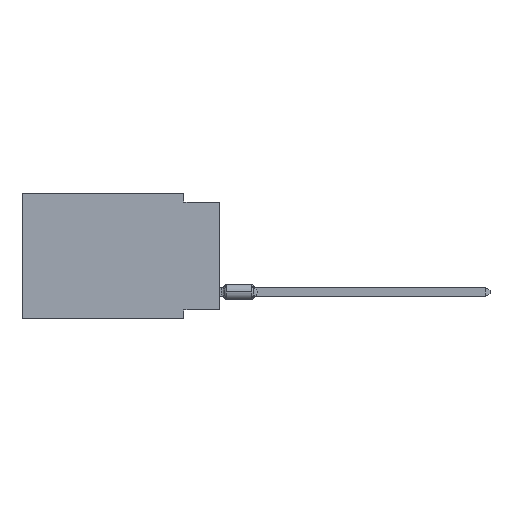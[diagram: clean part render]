
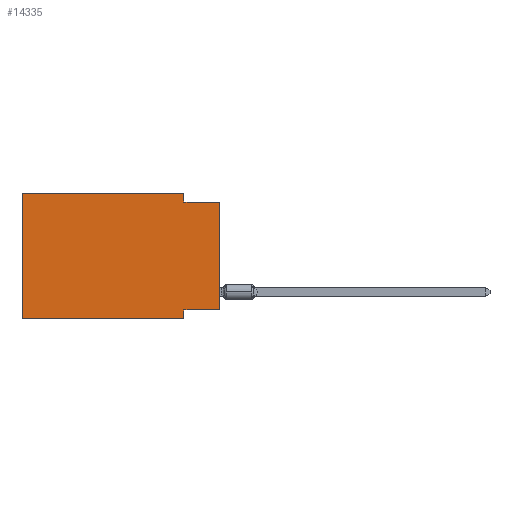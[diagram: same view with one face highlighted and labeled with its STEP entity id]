
A CAD part, left-side view. The second image highlights one B-rep face of the part: STEP entity #14335.
In plain terms, the highlighted planar face has unit normal (-1, 0, 0).
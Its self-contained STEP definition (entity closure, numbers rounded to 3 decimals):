
#148 = VECTOR ( 'NONE', #24377, 1000. ) ;
#185 = VECTOR ( 'NONE', #12506, 1000. ) ;
#1087 = DIRECTION ( 'NONE',  ( 1., 0., 0. ) ) ;
#1091 = ORIENTED_EDGE ( 'NONE', *, *, #11967, .F. ) ;
#1568 = EDGE_CURVE ( 'NONE', #18166, #24625, #8059, .T. ) ;
#1662 = ORIENTED_EDGE ( 'NONE', *, *, #21237, .T. ) ;
#1938 = ORIENTED_EDGE ( 'NONE', *, *, #7770, .F. ) ;
#2784 = CARTESIAN_POINT ( 'NONE',  ( 0., 2.54, 0. ) ) ;
#2973 = VERTEX_POINT ( 'NONE', #16576 ) ;
#4489 = VECTOR ( 'NONE', #13685, 1000. ) ;
#4841 = VERTEX_POINT ( 'NONE', #6124 ) ;
#5209 = LINE ( 'NONE', #14965, #17320 ) ;
#6124 = CARTESIAN_POINT ( 'NONE',  ( 0., 2.54, 0. ) ) ;
#6280 = CARTESIAN_POINT ( 'NONE',  ( 0., 0., -0.635 ) ) ;
#7612 = LINE ( 'NONE', #14299, #17727 ) ;
#7770 = EDGE_CURVE ( 'NONE', #19043, #13524, #5209, .T. ) ;
#7900 = LINE ( 'NONE', #15739, #4489 ) ;
#7977 = ORIENTED_EDGE ( 'NONE', *, *, #16869, .F. ) ;
#8059 = LINE ( 'NONE', #18111, #15852 ) ;
#8502 = ORIENTED_EDGE ( 'NONE', *, *, #1568, .F. ) ;
#8512 = DIRECTION ( 'NONE',  ( 0., -1., 0. ) ) ;
#8529 = LINE ( 'NONE', #24223, #185 ) ;
#8567 = CARTESIAN_POINT ( 'NONE',  ( 0., 13.97, -8.89 ) ) ;
#9347 = VERTEX_POINT ( 'NONE', #8567 ) ;
#9898 = CARTESIAN_POINT ( 'NONE',  ( 0., 2.54, -8.255 ) ) ;
#10142 = LINE ( 'NONE', #14255, #25301 ) ;
#10614 = DIRECTION ( 'NONE',  ( 0., 0., -1. ) ) ;
#11308 = ORIENTED_EDGE ( 'NONE', *, *, #21702, .T. ) ;
#11399 = EDGE_LOOP ( 'NONE', ( #1662, #1938, #12762, #7977, #1091, #11308, #14421, #8502 ) ) ;
#11967 = EDGE_CURVE ( 'NONE', #9347, #2973, #10142, .T. ) ;
#12386 = CARTESIAN_POINT ( 'NONE',  ( 0., 2.54, -8.89 ) ) ;
#12409 = LINE ( 'NONE', #2784, #12641 ) ;
#12506 = DIRECTION ( 'NONE',  ( 0., -1., 0. ) ) ;
#12641 = VECTOR ( 'NONE', #10614, 1000. ) ;
#12661 = CARTESIAN_POINT ( 'NONE',  ( 0., 0., 0. ) ) ;
#12762 = ORIENTED_EDGE ( 'NONE', *, *, #25180, .F. ) ;
#13092 = AXIS2_PLACEMENT_3D ( 'NONE', #22297, #1087, #20364 ) ;
#13524 = VERTEX_POINT ( 'NONE', #6280 ) ;
#13685 = DIRECTION ( 'NONE',  ( 0., 0., -1. ) ) ;
#13903 = EDGE_CURVE ( 'NONE', #24625, #21565, #7900, .T. ) ;
#14255 = CARTESIAN_POINT ( 'NONE',  ( 0., 13.97, 0. ) ) ;
#14299 = CARTESIAN_POINT ( 'NONE',  ( 0., 13.97, 0. ) ) ;
#14335 = ADVANCED_FACE ( 'NONE', ( #14447 ), #20620, .F. ) ;
#14421 = ORIENTED_EDGE ( 'NONE', *, *, #13903, .F. ) ;
#14447 = FACE_OUTER_BOUND ( 'NONE', #11399, .T. ) ;
#14965 = CARTESIAN_POINT ( 'NONE',  ( 0., 0., -0.635 ) ) ;
#15739 = CARTESIAN_POINT ( 'NONE',  ( 0., 2.54, -8.89 ) ) ;
#15852 = VECTOR ( 'NONE', #15911, 1000. ) ;
#15911 = DIRECTION ( 'NONE',  ( 0., 1., 0. ) ) ;
#16576 = CARTESIAN_POINT ( 'NONE',  ( 0., 13.97, 0. ) ) ;
#16785 = DIRECTION ( 'NONE',  ( 0., -1., 0. ) ) ;
#16869 = EDGE_CURVE ( 'NONE', #2973, #4841, #7612, .T. ) ;
#17320 = VECTOR ( 'NONE', #16785, 1000. ) ;
#17727 = VECTOR ( 'NONE', #8512, 1000. ) ;
#18111 = CARTESIAN_POINT ( 'NONE',  ( 0., 0., -8.255 ) ) ;
#18166 = VERTEX_POINT ( 'NONE', #21568 ) ;
#19043 = VERTEX_POINT ( 'NONE', #21263 ) ;
#19795 = DIRECTION ( 'NONE',  ( 0., 0., 1. ) ) ;
#20364 = DIRECTION ( 'NONE',  ( 0., 0., -1. ) ) ;
#20620 = PLANE ( 'NONE',  #13092 ) ;
#20646 = LINE ( 'NONE', #12661, #148 ) ;
#21237 = EDGE_CURVE ( 'NONE', #18166, #13524, #20646, .T. ) ;
#21263 = CARTESIAN_POINT ( 'NONE',  ( 0., 2.54, -0.635 ) ) ;
#21565 = VERTEX_POINT ( 'NONE', #12386 ) ;
#21568 = CARTESIAN_POINT ( 'NONE',  ( 0., 0., -8.255 ) ) ;
#21702 = EDGE_CURVE ( 'NONE', #9347, #21565, #8529, .T. ) ;
#22297 = CARTESIAN_POINT ( 'NONE',  ( 0., 13.97, 0. ) ) ;
#24223 = CARTESIAN_POINT ( 'NONE',  ( 0., 13.97, -8.89 ) ) ;
#24377 = DIRECTION ( 'NONE',  ( 0., 0., 1. ) ) ;
#24625 = VERTEX_POINT ( 'NONE', #9898 ) ;
#25180 = EDGE_CURVE ( 'NONE', #4841, #19043, #12409, .T. ) ;
#25301 = VECTOR ( 'NONE', #19795, 1000. ) ;
